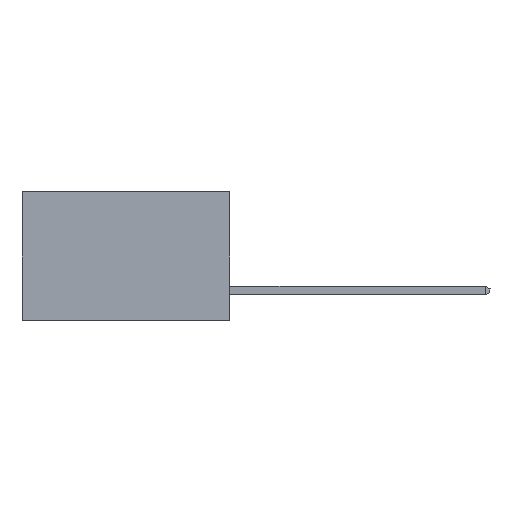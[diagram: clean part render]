
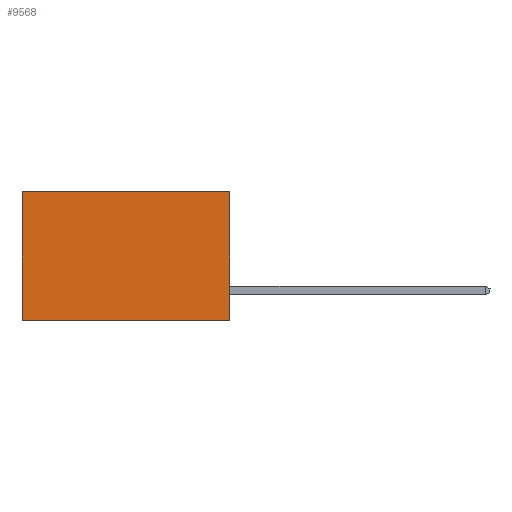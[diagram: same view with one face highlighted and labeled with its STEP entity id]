
A CAD part, left-side view. The second image highlights one B-rep face of the part: STEP entity #9568.
In plain terms, the highlighted planar face has unit normal (-1, 0, 0).
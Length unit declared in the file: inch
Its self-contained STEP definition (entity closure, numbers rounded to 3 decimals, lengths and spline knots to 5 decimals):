
#398 = AXIS2_PLACEMENT_3D ( 'NONE', #7135, #429, #10441 ) ;
#429 = DIRECTION ( 'NONE',  ( 1., 0., 0. ) ) ;
#2683 = VECTOR ( 'NONE', #18066, 39.37008 ) ;
#3452 = VERTEX_POINT ( 'NONE', #21638 ) ;
#3494 = EDGE_CURVE ( 'NONE', #18105, #3452, #9639, .T. ) ;
#4971 = DIRECTION ( 'NONE',  ( 0., 0., -1. ) ) ;
#5010 = VECTOR ( 'NONE', #4971, 39.37008 ) ;
#7032 = ORIENTED_EDGE ( 'NONE', *, *, #18204, .T. ) ;
#7135 = CARTESIAN_POINT ( 'NONE',  ( 0.2615, 0., -0.37 ) ) ;
#7279 = ORIENTED_EDGE ( 'NONE', *, *, #11504, .F. ) ;
#7670 = DIRECTION ( 'NONE',  ( 0., 0., -1. ) ) ;
#8567 = EDGE_CURVE ( 'NONE', #15615, #21049, #19228, .T. ) ;
#9568 = ADVANCED_FACE ( 'NONE', ( #17362 ), #12402, .F. ) ;
#9639 = LINE ( 'NONE', #13370, #5010 ) ;
#10441 = DIRECTION ( 'NONE',  ( 0., 0., -1. ) ) ;
#10486 = VECTOR ( 'NONE', #7670, 39.37008 ) ;
#10873 = CARTESIAN_POINT ( 'NONE',  ( 0.2615, 0.6, -0.37 ) ) ;
#11504 = EDGE_CURVE ( 'NONE', #3452, #21049, #14154, .T. ) ;
#11897 = CARTESIAN_POINT ( 'NONE',  ( 0.2615, 0.6, -0.37 ) ) ;
#12179 = CARTESIAN_POINT ( 'NONE',  ( 0.2615, 0., -0.37 ) ) ;
#12402 = PLANE ( 'NONE',  #398 ) ;
#13370 = CARTESIAN_POINT ( 'NONE',  ( 0.2615, 0., -0.37 ) ) ;
#14037 = DIRECTION ( 'NONE',  ( 0., 1., 0. ) ) ;
#14154 = LINE ( 'NONE', #12179, #14240 ) ;
#14240 = VECTOR ( 'NONE', #14037, 39.37008 ) ;
#14621 = CARTESIAN_POINT ( 'NONE',  ( 0.2615, 0.6, 0. ) ) ;
#14942 = ORIENTED_EDGE ( 'NONE', *, *, #3494, .F. ) ;
#15615 = VERTEX_POINT ( 'NONE', #14621 ) ;
#15822 = ORIENTED_EDGE ( 'NONE', *, *, #8567, .T. ) ;
#16287 = CARTESIAN_POINT ( 'NONE',  ( 0.2615, 0., 0. ) ) ;
#17133 = EDGE_LOOP ( 'NONE', ( #15822, #7279, #14942, #7032 ) ) ;
#17362 = FACE_OUTER_BOUND ( 'NONE', #17133, .T. ) ;
#17837 = CARTESIAN_POINT ( 'NONE',  ( 0.2615, 0., 0. ) ) ;
#18066 = DIRECTION ( 'NONE',  ( 0., 1., 0. ) ) ;
#18105 = VERTEX_POINT ( 'NONE', #17837 ) ;
#18183 = LINE ( 'NONE', #16287, #2683 ) ;
#18204 = EDGE_CURVE ( 'NONE', #18105, #15615, #18183, .T. ) ;
#19228 = LINE ( 'NONE', #10873, #10486 ) ;
#21049 = VERTEX_POINT ( 'NONE', #11897 ) ;
#21638 = CARTESIAN_POINT ( 'NONE',  ( 0.2615, 0., -0.37 ) ) ;
